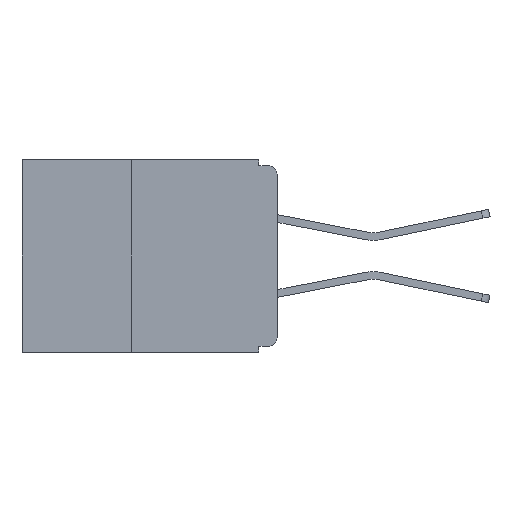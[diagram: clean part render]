
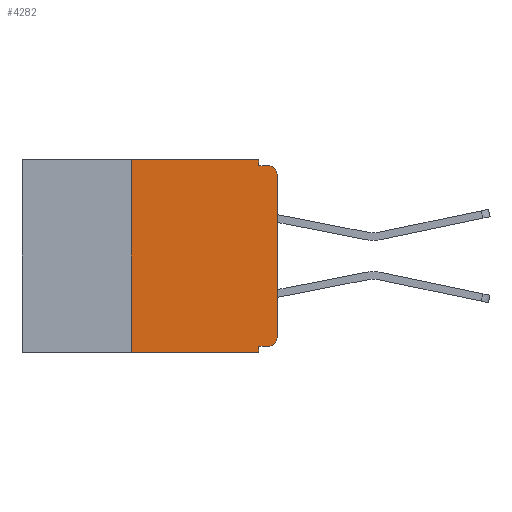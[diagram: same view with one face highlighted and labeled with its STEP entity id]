
A CAD part, left-side view. The second image highlights one B-rep face of the part: STEP entity #4282.
In plain terms, the highlighted planar face has unit normal (-1, 0, 0).
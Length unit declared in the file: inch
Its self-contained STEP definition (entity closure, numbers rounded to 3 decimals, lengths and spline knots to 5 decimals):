
#181 = AXIS2_PLACEMENT_3D ( 'NONE', #8954, #8671, #8563 ) ;
#536 = ORIENTED_EDGE ( 'NONE', *, *, #7500, .F. ) ;
#582 = CIRCLE ( 'NONE', #11533, 0.015 ) ;
#1052 = ORIENTED_EDGE ( 'NONE', *, *, #7127, .T. ) ;
#1242 = DIRECTION ( 'NONE',  ( 0., 0., 1. ) ) ;
#1618 = LINE ( 'NONE', #23234, #10228 ) ;
#1709 = DIRECTION ( 'NONE',  ( 0., 0., -1. ) ) ;
#1966 = LINE ( 'NONE', #14034, #20614 ) ;
#2122 = CARTESIAN_POINT ( 'NONE',  ( 0., 0.031, -0.01 ) ) ;
#2151 = CARTESIAN_POINT ( 'NONE',  ( 0., 0.031, 0. ) ) ;
#2275 = DIRECTION ( 'NONE',  ( -1., 0., 0. ) ) ;
#2612 = ORIENTED_EDGE ( 'NONE', *, *, #8819, .T. ) ;
#3045 = VERTEX_POINT ( 'NONE', #20083 ) ;
#3222 = EDGE_CURVE ( 'NONE', #15566, #16748, #21161, .T. ) ;
#3290 = VERTEX_POINT ( 'NONE', #13420 ) ;
#4139 = CARTESIAN_POINT ( 'NONE',  ( 0., 0., -0.32 ) ) ;
#4167 = CARTESIAN_POINT ( 'NONE',  ( 0., 0.031, -0.33 ) ) ;
#4282 = ADVANCED_FACE ( 'NONE', ( #11891 ), #17562, .F. ) ;
#4372 = CARTESIAN_POINT ( 'NONE',  ( 0., 0., -0.305 ) ) ;
#4488 = VECTOR ( 'NONE', #11894, 39.37008 ) ;
#4645 = EDGE_CURVE ( 'NONE', #17919, #10814, #22983, .T. ) ;
#5768 = ORIENTED_EDGE ( 'NONE', *, *, #21555, .F. ) ;
#5813 = CARTESIAN_POINT ( 'NONE',  ( 0., 0.25, -0.33 ) ) ;
#6079 = VECTOR ( 'NONE', #19170, 39.37008 ) ;
#6239 = CARTESIAN_POINT ( 'NONE',  ( 0., 0.015, -0.32 ) ) ;
#6287 = DIRECTION ( 'NONE',  ( 0., -1., 0. ) ) ;
#6860 = VECTOR ( 'NONE', #21859, 39.37008 ) ;
#7127 = EDGE_CURVE ( 'NONE', #16748, #3290, #582, .T. ) ;
#7213 = VERTEX_POINT ( 'NONE', #4167 ) ;
#7417 = ORIENTED_EDGE ( 'NONE', *, *, #15096, .F. ) ;
#7500 = EDGE_CURVE ( 'NONE', #3045, #7213, #11482, .T. ) ;
#7690 = ORIENTED_EDGE ( 'NONE', *, *, #16326, .F. ) ;
#8295 = ORIENTED_EDGE ( 'NONE', *, *, #15943, .T. ) ;
#8296 = CARTESIAN_POINT ( 'NONE',  ( 0., 0., -0.01 ) ) ;
#8563 = DIRECTION ( 'NONE',  ( 0., 0., -1. ) ) ;
#8578 = ORIENTED_EDGE ( 'NONE', *, *, #19511, .F. ) ;
#8671 = DIRECTION ( 'NONE',  ( -1., 0., 0. ) ) ;
#8819 = EDGE_CURVE ( 'NONE', #10483, #15566, #10842, .T. ) ;
#8954 = CARTESIAN_POINT ( 'NONE',  ( 0., 0.015, -0.305 ) ) ;
#9047 = VECTOR ( 'NONE', #16811, 39.37008 ) ;
#9577 = CARTESIAN_POINT ( 'NONE',  ( 0., 0., -0.025 ) ) ;
#10228 = VECTOR ( 'NONE', #10792, 39.37008 ) ;
#10483 = VERTEX_POINT ( 'NONE', #6239 ) ;
#10792 = DIRECTION ( 'NONE',  ( 0., -1., 0. ) ) ;
#10814 = VERTEX_POINT ( 'NONE', #2122 ) ;
#10842 = CIRCLE ( 'NONE', #181, 0.015 ) ;
#11133 = ORIENTED_EDGE ( 'NONE', *, *, #4645, .F. ) ;
#11482 = LINE ( 'NONE', #18456, #6079 ) ;
#11533 = AXIS2_PLACEMENT_3D ( 'NONE', #21799, #2275, #1709 ) ;
#11835 = EDGE_LOOP ( 'NONE', ( #22252, #1052, #7690, #11133, #7417, #8578, #8295, #536, #5768, #2612 ) ) ;
#11891 = FACE_OUTER_BOUND ( 'NONE', #11835, .T. ) ;
#11894 = DIRECTION ( 'NONE',  ( 0., 0., -1. ) ) ;
#11898 = CARTESIAN_POINT ( 'NONE',  ( 0., 0.031, 0. ) ) ;
#13420 = CARTESIAN_POINT ( 'NONE',  ( 0., 0.015, -0.01 ) ) ;
#14034 = CARTESIAN_POINT ( 'NONE',  ( 0., 0.25, -0.33 ) ) ;
#14629 = VECTOR ( 'NONE', #17235, 39.37008 ) ;
#15096 = EDGE_CURVE ( 'NONE', #18177, #17919, #22813, .T. ) ;
#15197 = LINE ( 'NONE', #8296, #14629 ) ;
#15566 = VERTEX_POINT ( 'NONE', #4372 ) ;
#15943 = EDGE_CURVE ( 'NONE', #19131, #7213, #1618, .T. ) ;
#16056 = LINE ( 'NONE', #4139, #9047 ) ;
#16326 = EDGE_CURVE ( 'NONE', #10814, #3290, #15197, .T. ) ;
#16748 = VERTEX_POINT ( 'NONE', #9577 ) ;
#16811 = DIRECTION ( 'NONE',  ( 0., 1., 0. ) ) ;
#16833 = AXIS2_PLACEMENT_3D ( 'NONE', #22269, #22274, #22876 ) ;
#17051 = CARTESIAN_POINT ( 'NONE',  ( 0., 0.437, 0. ) ) ;
#17235 = DIRECTION ( 'NONE',  ( 0., -1., 0. ) ) ;
#17562 = PLANE ( 'NONE',  #16833 ) ;
#17919 = VERTEX_POINT ( 'NONE', #2151 ) ;
#18177 = VERTEX_POINT ( 'NONE', #22699 ) ;
#18456 = CARTESIAN_POINT ( 'NONE',  ( 0., 0.031, -0.33 ) ) ;
#18639 = VECTOR ( 'NONE', #6287, 39.37008 ) ;
#19131 = VERTEX_POINT ( 'NONE', #5813 ) ;
#19170 = DIRECTION ( 'NONE',  ( 0., 0., -1. ) ) ;
#19511 = EDGE_CURVE ( 'NONE', #19131, #18177, #1966, .T. ) ;
#20083 = CARTESIAN_POINT ( 'NONE',  ( 0., 0.031, -0.32 ) ) ;
#20614 = VECTOR ( 'NONE', #1242, 39.37008 ) ;
#21037 = CARTESIAN_POINT ( 'NONE',  ( 0., 0., 0. ) ) ;
#21161 = LINE ( 'NONE', #21037, #6860 ) ;
#21555 = EDGE_CURVE ( 'NONE', #10483, #3045, #16056, .T. ) ;
#21799 = CARTESIAN_POINT ( 'NONE',  ( 0., 0.015, -0.025 ) ) ;
#21859 = DIRECTION ( 'NONE',  ( 0., 0., 1. ) ) ;
#22252 = ORIENTED_EDGE ( 'NONE', *, *, #3222, .T. ) ;
#22269 = CARTESIAN_POINT ( 'NONE',  ( 0., 0.437, 0. ) ) ;
#22274 = DIRECTION ( 'NONE',  ( 1., 0., 0. ) ) ;
#22699 = CARTESIAN_POINT ( 'NONE',  ( 0., 0.25, 0. ) ) ;
#22813 = LINE ( 'NONE', #17051, #18639 ) ;
#22876 = DIRECTION ( 'NONE',  ( 0., 0., -1. ) ) ;
#22983 = LINE ( 'NONE', #11898, #4488 ) ;
#23234 = CARTESIAN_POINT ( 'NONE',  ( 0., 0.437, -0.33 ) ) ;
